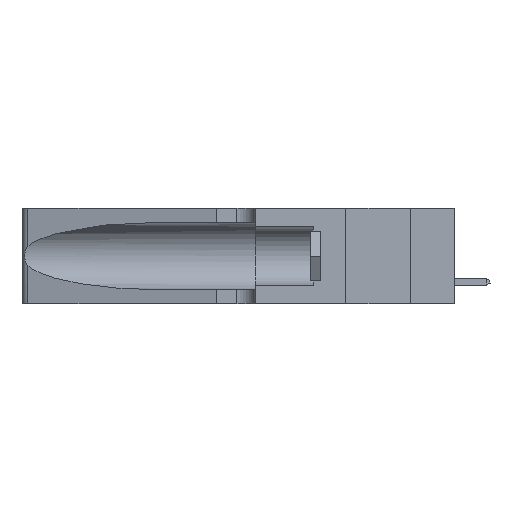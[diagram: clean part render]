
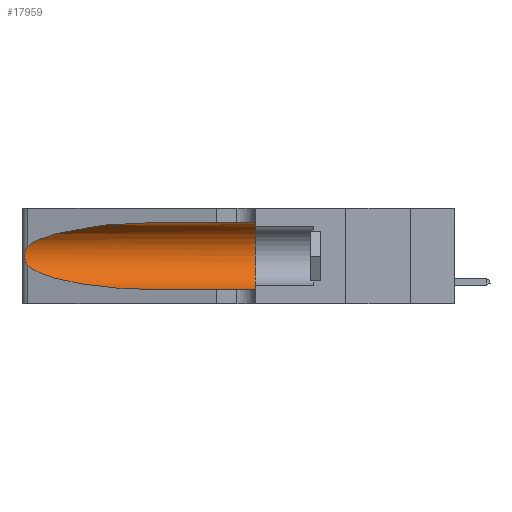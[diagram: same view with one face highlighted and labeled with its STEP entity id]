
A CAD part, left-side view. The second image highlights one B-rep face of the part: STEP entity #17959.
In plain terms, the highlighted cylindrical face has radius 3.308 mm (diameter 6.617 mm), a partial arc.
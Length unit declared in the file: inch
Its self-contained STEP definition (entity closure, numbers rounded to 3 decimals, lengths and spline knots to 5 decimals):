
#75 = DIRECTION ( 'NONE',  ( 0., -1., 0. ) ) ;
#573 = EDGE_CURVE ( 'NONE', #20753, #14967, #4148, .T. ) ;
#1283 = CARTESIAN_POINT ( 'NONE',  ( 0.25487, 1.22718, 0.22369 ) ) ;
#1735 = CARTESIAN_POINT ( 'NONE',  ( 0.25555, 1.22994, 0.2215 ) ) ;
#1813 = CARTESIAN_POINT ( 'NONE',  ( 0.26017, 1.23833, 0.17102 ) ) ;
#2381 = CARTESIAN_POINT ( 'NONE',  ( 0.1305, 0.72297, 0.05475 ) ) ;
#2421 = CIRCLE ( 'NONE', #16638, 0.13025 ) ;
#2692 = FACE_OUTER_BOUND ( 'NONE', #11935, .T. ) ;
#3166 = CARTESIAN_POINT ( 'NONE',  ( 0.1305, 1.61858, 0.05475 ) ) ;
#3383 = EDGE_CURVE ( 'NONE', #21358, #20753, #16868, .T. ) ;
#3788 = CARTESIAN_POINT ( 'NONE',  ( 0.25487, 1.22718, 0.14631 ) ) ;
#4148 =( BOUNDED_CURVE ( )  B_SPLINE_CURVE ( 3, ( #16441, #4577, #10493, #2381 ),
 .UNSPECIFIED., .F., .F. ) 
 B_SPLINE_CURVE_WITH_KNOTS ( ( 4, 4 ),
 ( 3.44316, 4.71239 ),
 .UNSPECIFIED. ) 
 CURVE ( )  GEOMETRIC_REPRESENTATION_ITEM ( )  RATIONAL_B_SPLINE_CURVE ( ( 1., 0.87, 0.87, 1. ) ) 
 REPRESENTATION_ITEM ( '' )  );
#4214 = CARTESIAN_POINT ( 'NONE',  ( 0.25487, 1.22718, 0.22369 ) ) ;
#4256 = VERTEX_POINT ( 'NONE', #6251 ) ;
#4577 = CARTESIAN_POINT ( 'NONE',  ( 0.2373, 1.15595, 0.08982 ) ) ;
#5812 = EDGE_CURVE ( 'NONE', #14967, #23683, #24033, .T. ) ;
#5862 = CARTESIAN_POINT ( 'NONE',  ( 0.25854, 1.2359, 0.20912 ) ) ;
#6011 = EDGE_CURVE ( 'NONE', #25889, #21358, #7567, .T. ) ;
#6149 = CYLINDRICAL_SURFACE ( 'NONE', #18658, 0.13025 ) ;
#6251 = CARTESIAN_POINT ( 'NONE',  ( 0.1305, 0.35, 0.31525 ) ) ;
#6408 = CARTESIAN_POINT ( 'NONE',  ( 0.1305, 0.35, 0.05475 ) ) ;
#6736 = CARTESIAN_POINT ( 'NONE',  ( 0.1305, 0.72297, 0.05475 ) ) ;
#6934 = ORIENTED_EDGE ( 'NONE', *, *, #6011, .T. ) ;
#7567 =( BOUNDED_CURVE ( )  B_SPLINE_CURVE ( 3, ( #25626, #7762, #12065, #4214 ),
 .UNSPECIFIED., .F., .T. ) 
 B_SPLINE_CURVE_WITH_KNOTS ( ( 4, 4 ),
 ( 1.5708, 2.84003 ),
 .UNSPECIFIED. ) 
 CURVE ( )  GEOMETRIC_REPRESENTATION_ITEM ( )  RATIONAL_B_SPLINE_CURVE ( ( 1., 0.87, 0.87, 1. ) ) 
 REPRESENTATION_ITEM ( '' )  );
#7762 = CARTESIAN_POINT ( 'NONE',  ( 0.18966, 0.96281, 0.31525 ) ) ;
#7819 = CARTESIAN_POINT ( 'NONE',  ( 0.25487, 1.22718, 0.22369 ) ) ;
#7910 = CARTESIAN_POINT ( 'NONE',  ( 0.25639, 1.23186, 0.15144 ) ) ;
#9357 = DIRECTION ( 'NONE',  ( 0., -1., 0. ) ) ;
#9933 = CARTESIAN_POINT ( 'NONE',  ( 0.25487, 1.22718, 0.14631 ) ) ;
#10118 = CARTESIAN_POINT ( 'NONE',  ( 0.1305, 1.61858, 0.185 ) ) ;
#10386 = DIRECTION ( 'NONE',  ( 0., 1., 0. ) ) ;
#10493 = CARTESIAN_POINT ( 'NONE',  ( 0.18966, 0.96281, 0.05475 ) ) ;
#10829 = VECTOR ( 'NONE', #16924, 39.37008 ) ;
#11732 = ORIENTED_EDGE ( 'NONE', *, *, #3383, .T. ) ;
#11884 = CARTESIAN_POINT ( 'NONE',  ( 0.26075, 1.23896, 0.19203 ) ) ;
#11935 = EDGE_LOOP ( 'NONE', ( #6934, #11732, #22899, #19855, #14557, #20434 ) ) ;
#11965 = CARTESIAN_POINT ( 'NONE',  ( 0.25789, 1.23486, 0.15765 ) ) ;
#12058 = EDGE_CURVE ( 'NONE', #25889, #4256, #22656, .T. ) ;
#12065 = CARTESIAN_POINT ( 'NONE',  ( 0.2373, 1.15595, 0.28018 ) ) ;
#13458 = CARTESIAN_POINT ( 'NONE',  ( 0.1305, 0.72297, 0.31525 ) ) ;
#13884 = DIRECTION ( 'NONE',  ( 0., 0., -1. ) ) ;
#14066 = DIRECTION ( 'NONE',  ( 0., 0., 1. ) ) ;
#14557 = ORIENTED_EDGE ( 'NONE', *, *, #17100, .F. ) ;
#14967 = VERTEX_POINT ( 'NONE', #6736 ) ;
#15970 = CARTESIAN_POINT ( 'NONE',  ( 0.26075, 1.23896, 0.178 ) ) ;
#16441 = CARTESIAN_POINT ( 'NONE',  ( 0.25487, 1.22718, 0.14631 ) ) ;
#16638 = AXIS2_PLACEMENT_3D ( 'NONE', #20249, #10386, #14066 ) ;
#16868 = B_SPLINE_CURVE_WITH_KNOTS ( 'NONE', 3,
 ( #7819, #1735, #18056, #19983, #5862, #19813, #11884, #15970, #1813, #22054, #11965, #7910, #21891, #9933 ),
 .UNSPECIFIED., .F., .F.,
 ( 4, 2, 2, 2, 2, 2, 4 ),
 ( 0., 0.00027, 0.00053, 0.00107, 0.0016, 0.00187, 0.00214 ),
 .UNSPECIFIED. ) ;
#16924 = DIRECTION ( 'NONE',  ( 0., -1., 0. ) ) ;
#17100 = EDGE_CURVE ( 'NONE', #4256, #23683, #2421, .T. ) ;
#17959 = ADVANCED_FACE ( 'NONE', ( #2692 ), #6149, .F. ) ;
#18056 = CARTESIAN_POINT ( 'NONE',  ( 0.25639, 1.23184, 0.21858 ) ) ;
#18658 = AXIS2_PLACEMENT_3D ( 'NONE', #10118, #75, #13884 ) ;
#19109 = CARTESIAN_POINT ( 'NONE',  ( 0.1305, 1.61858, 0.31525 ) ) ;
#19813 = CARTESIAN_POINT ( 'NONE',  ( 0.26018, 1.23835, 0.19895 ) ) ;
#19855 = ORIENTED_EDGE ( 'NONE', *, *, #5812, .T. ) ;
#19983 = CARTESIAN_POINT ( 'NONE',  ( 0.25787, 1.23484, 0.2124 ) ) ;
#20249 = CARTESIAN_POINT ( 'NONE',  ( 0.1305, 0.35, 0.185 ) ) ;
#20434 = ORIENTED_EDGE ( 'NONE', *, *, #12058, .F. ) ;
#20753 = VERTEX_POINT ( 'NONE', #3788 ) ;
#21358 = VERTEX_POINT ( 'NONE', #1283 ) ;
#21891 = CARTESIAN_POINT ( 'NONE',  ( 0.25555, 1.22993, 0.14849 ) ) ;
#22054 = CARTESIAN_POINT ( 'NONE',  ( 0.25856, 1.23593, 0.16098 ) ) ;
#22656 = LINE ( 'NONE', #19109, #10829 ) ;
#22775 = VECTOR ( 'NONE', #9357, 39.37008 ) ;
#22899 = ORIENTED_EDGE ( 'NONE', *, *, #573, .T. ) ;
#23683 = VERTEX_POINT ( 'NONE', #6408 ) ;
#24033 = LINE ( 'NONE', #3166, #22775 ) ;
#25626 = CARTESIAN_POINT ( 'NONE',  ( 0.1305, 0.72297, 0.31525 ) ) ;
#25889 = VERTEX_POINT ( 'NONE', #13458 ) ;
